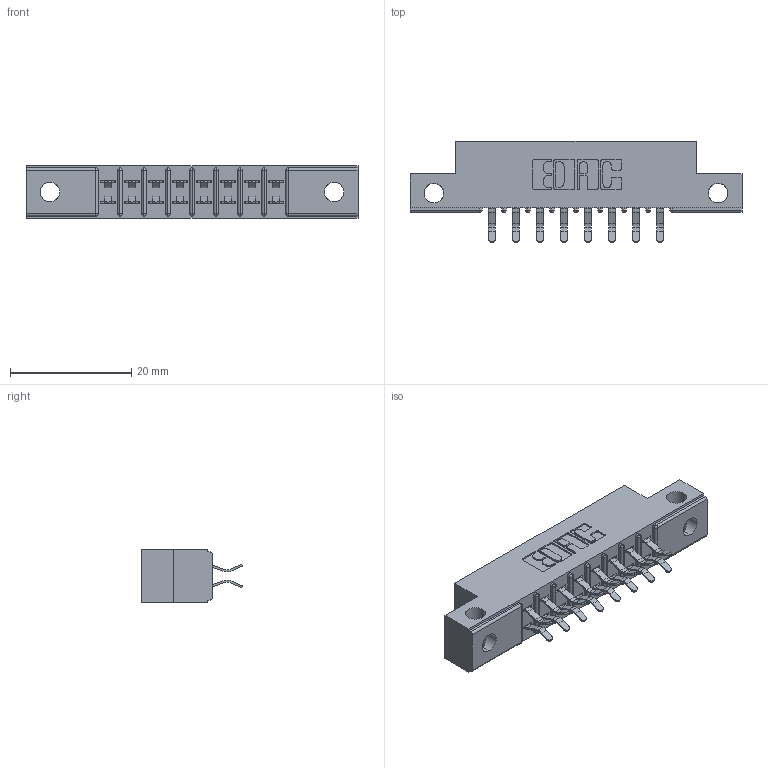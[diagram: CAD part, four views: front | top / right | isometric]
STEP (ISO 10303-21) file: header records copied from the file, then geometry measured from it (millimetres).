
FILE_DESCRIPTION (( 'STEP AP203' ), '1' );
FILE_NAME ('305-016-556-512.STEP', '2020-09-19T20:33:07', ( '' ), ( '' ), 'SwSTEP 2.0', 'SolidWorks 2020', '' );
FILE_SCHEMA (( 'CONFIG_CONTROL_DESIGN' ));
Length unit declared in the file: inch
Products named in the file (3): 305-016-556-512; 305 Part_.128 Dia; 305-290-001_556
Assembly tree (17 placements, depth 2):
  305-016-556-512
    305 Part_.128 Dia
    305-290-001_556  x16
Bounding box: 54.71 x 16.64 x 8.71 mm (x, y, z)
Volume: 3195.9 mm3; surface area: 5485.2 mm2
Topology: 17 solids, 17 shells, 1024 faces, 2936 edges, 1908 vertices
Faces by surface type: plane 564, cylinder 428, sphere 32
Entity records: 13429 total; most frequent: CARTESIAN_POINT 2274, ORIENTED_EDGE 2208, DIRECTION 2170, EDGE_CURVE 1104, VECTOR 834, LINE 834, VERTEX_POINT 708, AXIS2_PLACEMENT_3D 668
